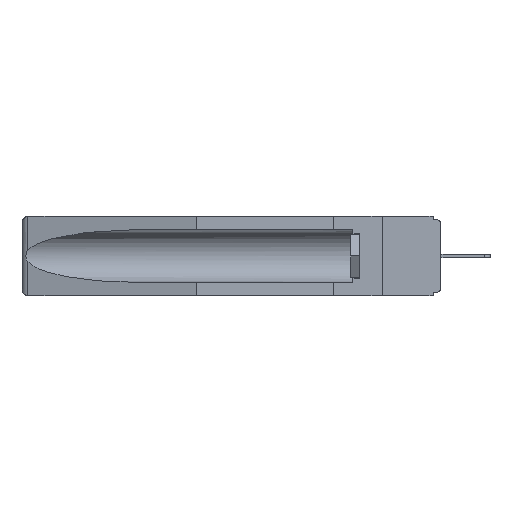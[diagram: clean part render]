
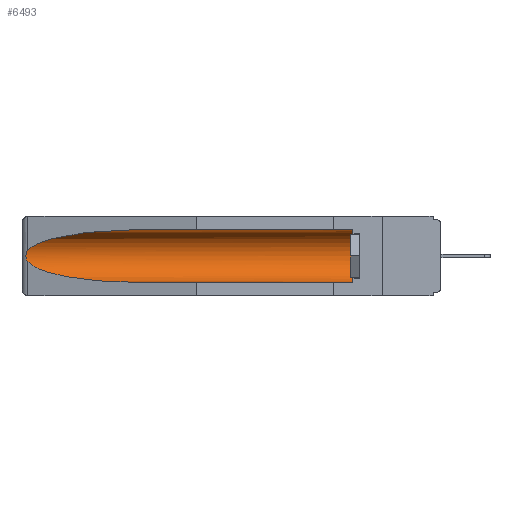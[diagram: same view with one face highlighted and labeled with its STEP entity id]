
A CAD part, left-side view. The second image highlights one B-rep face of the part: STEP entity #6493.
In plain terms, the highlighted cylindrical face has radius 2.857 mm (diameter 5.715 mm), a partial arc.
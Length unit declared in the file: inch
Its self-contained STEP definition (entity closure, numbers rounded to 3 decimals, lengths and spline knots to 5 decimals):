
#187 = LINE ( 'NONE', #7157, #3576 ) ;
#688 = EDGE_CURVE ( 'NONE', #14472, #10660, #10756, .T. ) ;
#1095 = CARTESIAN_POINT ( 'NONE',  ( 0.155, 1.07973, -0.284 ) ) ;
#1515 = EDGE_CURVE ( 'NONE', #10660, #11431, #2983, .T. ) ;
#1578 = ORIENTED_EDGE ( 'NONE', *, *, #11444, .T. ) ;
#2305 = CARTESIAN_POINT ( 'NONE',  ( 0.26537, 1.52718, -0.14972 ) ) ;
#2580 = DIRECTION ( 'NONE',  ( 0., 0., 1. ) ) ;
#2983 =( BOUNDED_CURVE ( )  B_SPLINE_CURVE ( 3, ( #13357, #10170, #13700, #14048 ),
 .UNSPECIFIED., .F., .F. ) 
 B_SPLINE_CURVE_WITH_KNOTS ( ( 4, 4 ),
 ( 4.71239, 6.08839 ),
 .UNSPECIFIED. ) 
 CURVE ( )  GEOMETRIC_REPRESENTATION_ITEM ( )  RATIONAL_B_SPLINE_CURVE ( ( 1., 0.848, 0.848, 1. ) ) 
 REPRESENTATION_ITEM ( '' )  );
#3555 = CIRCLE ( 'NONE', #13087, 0.1125 ) ;
#3576 = VECTOR ( 'NONE', #8601, 39.37008 ) ;
#3731 = CARTESIAN_POINT ( 'NONE',  ( 0.26654, 1.53092, -0.15636 ) ) ;
#3754 = DIRECTION ( 'NONE',  ( 0., 0., 1. ) ) ;
#3832 = VERTEX_POINT ( 'NONE', #6135 ) ;
#3846 = DIRECTION ( 'NONE',  ( 0., -1., 0. ) ) ;
#5028 = EDGE_CURVE ( 'NONE', #8466, #14472, #3555, .T. ) ;
#5151 = CARTESIAN_POINT ( 'NONE',  ( 0.2675, 1.53308, -0.16763 ) ) ;
#5165 = VERTEX_POINT ( 'NONE', #1095 ) ;
#5520 = B_SPLINE_CURVE_WITH_KNOTS ( 'NONE', 3,
 ( #2305, #12181, #3731, #13595, #5151, #15026, #6589, #16430, #8008, #17801 ),
 .UNSPECIFIED., .F., .F.,
 ( 4, 2, 2, 2, 4 ),
 ( 0., 0.00029, 0.00058, 0.00087, 0.00117 ),
 .UNSPECIFIED. ) ;
#5808 = ORIENTED_EDGE ( 'NONE', *, *, #11405, .T. ) ;
#6135 = CARTESIAN_POINT ( 'NONE',  ( 0.26537, 1.52718, -0.19328 ) ) ;
#6493 = ADVANCED_FACE ( 'NONE', ( #16298 ), #8828, .F. ) ;
#6589 = CARTESIAN_POINT ( 'NONE',  ( 0.2673, 1.53269, -0.17917 ) ) ;
#6844 = DIRECTION ( 'NONE',  ( 0., 1., 0. ) ) ;
#7157 = CARTESIAN_POINT ( 'NONE',  ( 0.155, -0.30754, -0.284 ) ) ;
#8008 = CARTESIAN_POINT ( 'NONE',  ( 0.26597, 1.5296, -0.19026 ) ) ;
#8466 = VERTEX_POINT ( 'NONE', #10114 ) ;
#8601 = DIRECTION ( 'NONE',  ( 0., 1., 0. ) ) ;
#8828 = CYLINDRICAL_SURFACE ( 'NONE', #11003, 0.1125 ) ;
#9332 = CARTESIAN_POINT ( 'NONE',  ( 0.155, 1.07973, -0.284 ) ) ;
#9589 = ORIENTED_EDGE ( 'NONE', *, *, #14925, .F. ) ;
#10025 = ORIENTED_EDGE ( 'NONE', *, *, #688, .T. ) ;
#10114 = CARTESIAN_POINT ( 'NONE',  ( 0.155, 0.126, -0.284 ) ) ;
#10170 = CARTESIAN_POINT ( 'NONE',  ( 0.21114, 1.30732, -0.059 ) ) ;
#10660 = VERTEX_POINT ( 'NONE', #17658 ) ;
#10756 = LINE ( 'NONE', #15005, #17743 ) ;
#10790 = CARTESIAN_POINT ( 'NONE',  ( 0.26537, 1.52718, -0.14972 ) ) ;
#11003 = AXIS2_PLACEMENT_3D ( 'NONE', #12446, #6844, #2580 ) ;
#11405 = EDGE_CURVE ( 'NONE', #3832, #5165, #16530, .T. ) ;
#11431 = VERTEX_POINT ( 'NONE', #10790 ) ;
#11444 = EDGE_CURVE ( 'NONE', #11431, #3832, #5520, .T. ) ;
#12181 = CARTESIAN_POINT ( 'NONE',  ( 0.26597, 1.52961, -0.15275 ) ) ;
#12446 = CARTESIAN_POINT ( 'NONE',  ( 0.155, -0.30754, -0.1715 ) ) ;
#13087 = AXIS2_PLACEMENT_3D ( 'NONE', #15603, #3846, #3754 ) ;
#13357 = CARTESIAN_POINT ( 'NONE',  ( 0.155, 1.07973, -0.059 ) ) ;
#13595 = CARTESIAN_POINT ( 'NONE',  ( 0.2673, 1.5327, -0.16383 ) ) ;
#13700 = CARTESIAN_POINT ( 'NONE',  ( 0.25451, 1.48313, -0.09465 ) ) ;
#14048 = CARTESIAN_POINT ( 'NONE',  ( 0.26537, 1.52718, -0.14972 ) ) ;
#14472 = VERTEX_POINT ( 'NONE', #17372 ) ;
#14905 = CARTESIAN_POINT ( 'NONE',  ( 0.25451, 1.48313, -0.24835 ) ) ;
#14925 = EDGE_CURVE ( 'NONE', #8466, #5165, #187, .T. ) ;
#15005 = CARTESIAN_POINT ( 'NONE',  ( 0.155, -0.30754, -0.059 ) ) ;
#15026 = CARTESIAN_POINT ( 'NONE',  ( 0.2675, 1.53308, -0.17534 ) ) ;
#15603 = CARTESIAN_POINT ( 'NONE',  ( 0.155, 0.126, -0.1715 ) ) ;
#16160 = ORIENTED_EDGE ( 'NONE', *, *, #1515, .T. ) ;
#16298 = FACE_OUTER_BOUND ( 'NONE', #18088, .T. ) ;
#16311 = CARTESIAN_POINT ( 'NONE',  ( 0.26537, 1.52718, -0.19328 ) ) ;
#16430 = CARTESIAN_POINT ( 'NONE',  ( 0.26655, 1.53094, -0.18657 ) ) ;
#16530 =( BOUNDED_CURVE ( )  B_SPLINE_CURVE ( 3, ( #16311, #14905, #17685, #9332 ),
 .UNSPECIFIED., .F., .F. ) 
 B_SPLINE_CURVE_WITH_KNOTS ( ( 4, 4 ),
 ( 0.1948, 1.5708 ),
 .UNSPECIFIED. ) 
 CURVE ( )  GEOMETRIC_REPRESENTATION_ITEM ( )  RATIONAL_B_SPLINE_CURVE ( ( 1., 0.848, 0.848, 1. ) ) 
 REPRESENTATION_ITEM ( '' )  );
#17036 = ORIENTED_EDGE ( 'NONE', *, *, #5028, .T. ) ;
#17372 = CARTESIAN_POINT ( 'NONE',  ( 0.155, 0.126, -0.059 ) ) ;
#17658 = CARTESIAN_POINT ( 'NONE',  ( 0.155, 1.07973, -0.059 ) ) ;
#17685 = CARTESIAN_POINT ( 'NONE',  ( 0.21114, 1.30732, -0.284 ) ) ;
#17743 = VECTOR ( 'NONE', #17798, 39.37008 ) ;
#17798 = DIRECTION ( 'NONE',  ( 0., 1., 0. ) ) ;
#17801 = CARTESIAN_POINT ( 'NONE',  ( 0.26537, 1.52718, -0.19328 ) ) ;
#18088 = EDGE_LOOP ( 'NONE', ( #16160, #1578, #5808, #9589, #17036, #10025 ) ) ;
